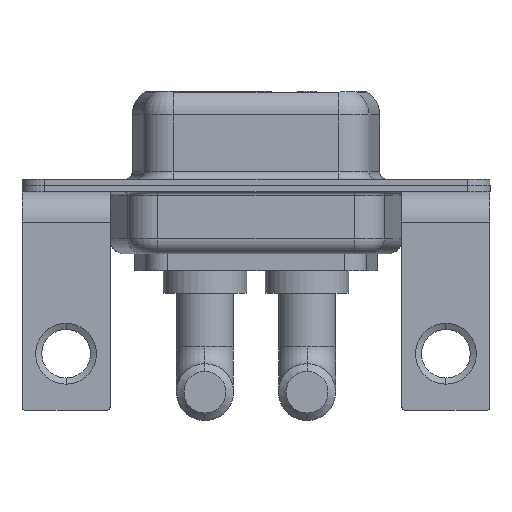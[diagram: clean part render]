
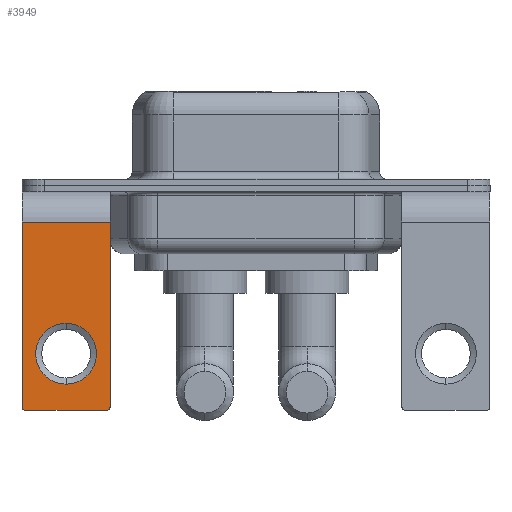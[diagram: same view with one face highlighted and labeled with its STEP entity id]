
A CAD part, front view. The second image highlights one B-rep face of the part: STEP entity #3949.
In plain terms, the highlighted planar face has unit normal (0, -1, 0).
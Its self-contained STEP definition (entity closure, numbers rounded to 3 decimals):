
#174 = EDGE_CURVE ( 'NONE', #8319, #3312, #5607, .T. ) ;
#270 = ORIENTED_EDGE ( 'NONE', *, *, #3873, .T. ) ;
#393 = DIRECTION ( 'NONE',  ( 0., 1., 0. ) ) ;
#467 = EDGE_CURVE ( 'NONE', #1125, #4903, #8653, .T. ) ;
#614 = VECTOR ( 'NONE', #7621, 1000. ) ;
#725 = ORIENTED_EDGE ( 'NONE', *, *, #4298, .T. ) ;
#876 = ORIENTED_EDGE ( 'NONE', *, *, #7340, .T. ) ;
#1038 = DIRECTION ( 'NONE',  ( -1., 0., 0. ) ) ;
#1125 = VERTEX_POINT ( 'NONE', #11932 ) ;
#1298 = ORIENTED_EDGE ( 'NONE', *, *, #467, .F. ) ;
#1575 = DIRECTION ( 'NONE',  ( 0., 1., 0. ) ) ;
#1897 = EDGE_CURVE ( 'NONE', #8978, #12064, #12141, .T. ) ;
#1961 = DIRECTION ( 'NONE',  ( 0., -1., 0. ) ) ;
#2338 = AXIS2_PLACEMENT_3D ( 'NONE', #7494, #13983, #10568 ) ;
#2530 = FACE_OUTER_BOUND ( 'NONE', #5943, .T. ) ;
#3092 = LINE ( 'NONE', #9731, #13805 ) ;
#3312 = VERTEX_POINT ( 'NONE', #8552 ) ;
#3322 = CARTESIAN_POINT ( 'NONE',  ( -2.65, -6.25, -14.55 ) ) ;
#3490 = AXIS2_PLACEMENT_3D ( 'NONE', #9381, #6243, #13793 ) ;
#3873 = EDGE_CURVE ( 'NONE', #13161, #4903, #11270, .T. ) ;
#3949 = ADVANCED_FACE ( 'NONE', ( #7955, #2530 ), #5549, .F. ) ;
#4248 = DIRECTION ( 'NONE',  ( -1., 0., 0. ) ) ;
#4298 = EDGE_CURVE ( 'NONE', #8319, #5738, #3092, .T. ) ;
#4460 = AXIS2_PLACEMENT_3D ( 'NONE', #3322, #1961, #8947 ) ;
#4903 = VERTEX_POINT ( 'NONE', #9863 ) ;
#5147 = ORIENTED_EDGE ( 'NONE', *, *, #1897, .T. ) ;
#5284 = CIRCLE ( 'NONE', #8223, 2. ) ;
#5549 = PLANE ( 'NONE',  #8556 ) ;
#5607 = LINE ( 'NONE', #6945, #6604 ) ;
#5738 = VERTEX_POINT ( 'NONE', #9148 ) ;
#5943 = EDGE_LOOP ( 'NONE', ( #7361, #270, #1298, #8901, #10560, #725 ) ) ;
#6243 = DIRECTION ( 'NONE',  ( 0., 1., 0. ) ) ;
#6604 = VECTOR ( 'NONE', #9017, 1000. ) ;
#6831 = EDGE_CURVE ( 'NONE', #5738, #13161, #8608, .T. ) ;
#6906 = EDGE_LOOP ( 'NONE', ( #876, #5147 ) ) ;
#6945 = CARTESIAN_POINT ( 'NONE',  ( 2.9, -6.25, -2.4 ) ) ;
#7115 = CIRCLE ( 'NONE', #2338, 0.25 ) ;
#7137 = CARTESIAN_POINT ( 'NONE',  ( 0., -6.25, -11.07 ) ) ;
#7340 = EDGE_CURVE ( 'NONE', #12064, #8978, #5284, .T. ) ;
#7361 = ORIENTED_EDGE ( 'NONE', *, *, #6831, .T. ) ;
#7494 = CARTESIAN_POINT ( 'NONE',  ( 2.65, -6.25, -14.55 ) ) ;
#7517 = EDGE_CURVE ( 'NONE', #1125, #3312, #7115, .T. ) ;
#7621 = DIRECTION ( 'NONE',  ( 0., 0., -1. ) ) ;
#7955 = FACE_BOUND ( 'NONE', #6906, .T. ) ;
#8223 = AXIS2_PLACEMENT_3D ( 'NONE', #7137, #1575, #11406 ) ;
#8319 = VERTEX_POINT ( 'NONE', #11370 ) ;
#8552 = CARTESIAN_POINT ( 'NONE',  ( 2.9, -6.25, -14.55 ) ) ;
#8556 = AXIS2_PLACEMENT_3D ( 'NONE', #9897, #393, #12297 ) ;
#8608 = LINE ( 'NONE', #10829, #614 ) ;
#8653 = LINE ( 'NONE', #10731, #10038 ) ;
#8901 = ORIENTED_EDGE ( 'NONE', *, *, #7517, .T. ) ;
#8947 = DIRECTION ( 'NONE',  ( 0., 0., 1. ) ) ;
#8978 = VERTEX_POINT ( 'NONE', #13636 ) ;
#9017 = DIRECTION ( 'NONE',  ( 0., 0., -1. ) ) ;
#9148 = CARTESIAN_POINT ( 'NONE',  ( -2.9, -6.25, -2.4 ) ) ;
#9381 = CARTESIAN_POINT ( 'NONE',  ( 0., -6.25, -11.07 ) ) ;
#9731 = CARTESIAN_POINT ( 'NONE',  ( 2.9, -6.25, -2.4 ) ) ;
#9863 = CARTESIAN_POINT ( 'NONE',  ( -2.65, -6.25, -14.8 ) ) ;
#9897 = CARTESIAN_POINT ( 'NONE',  ( 2.9, -6.25, -2.4 ) ) ;
#10038 = VECTOR ( 'NONE', #1038, 1000. ) ;
#10560 = ORIENTED_EDGE ( 'NONE', *, *, #174, .F. ) ;
#10568 = DIRECTION ( 'NONE',  ( 0., 0., 1. ) ) ;
#10731 = CARTESIAN_POINT ( 'NONE',  ( 2.9, -6.25, -14.8 ) ) ;
#10829 = CARTESIAN_POINT ( 'NONE',  ( -2.9, -6.25, -2.4 ) ) ;
#11270 = CIRCLE ( 'NONE', #4460, 0.25 ) ;
#11370 = CARTESIAN_POINT ( 'NONE',  ( 2.9, -6.25, -2.4 ) ) ;
#11406 = DIRECTION ( 'NONE',  ( 0., 0., 1. ) ) ;
#11932 = CARTESIAN_POINT ( 'NONE',  ( 2.65, -6.25, -14.8 ) ) ;
#12064 = VERTEX_POINT ( 'NONE', #12497 ) ;
#12141 = CIRCLE ( 'NONE', #3490, 2. ) ;
#12297 = DIRECTION ( 'NONE',  ( 0., 0., 1. ) ) ;
#12497 = CARTESIAN_POINT ( 'NONE',  ( 0., -6.25, -13.07 ) ) ;
#12621 = CARTESIAN_POINT ( 'NONE',  ( -2.9, -6.25, -14.55 ) ) ;
#13161 = VERTEX_POINT ( 'NONE', #12621 ) ;
#13636 = CARTESIAN_POINT ( 'NONE',  ( 0., -6.25, -9.07 ) ) ;
#13793 = DIRECTION ( 'NONE',  ( 0., 0., 1. ) ) ;
#13805 = VECTOR ( 'NONE', #4248, 1000. ) ;
#13983 = DIRECTION ( 'NONE',  ( 0., -1., 0. ) ) ;
